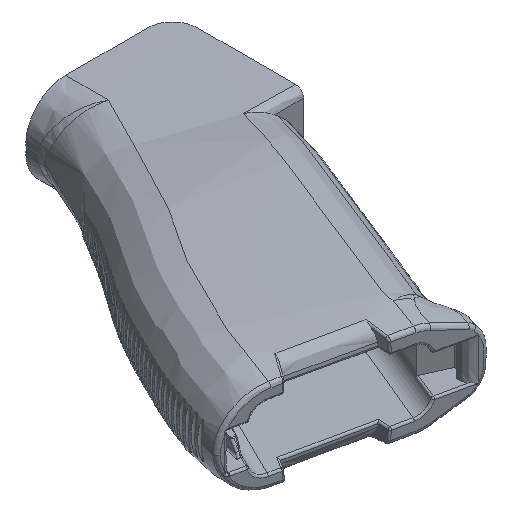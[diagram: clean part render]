
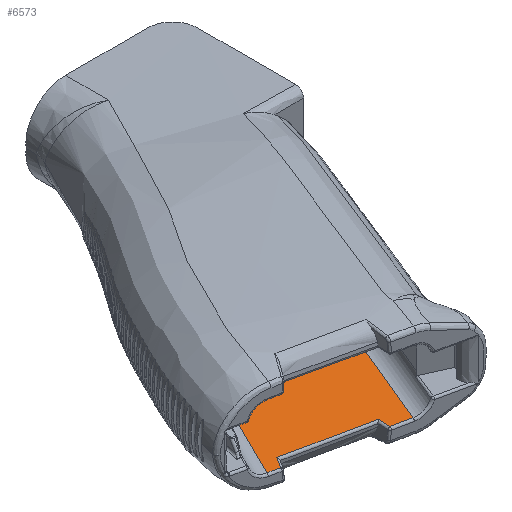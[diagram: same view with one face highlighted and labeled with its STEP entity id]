
A CAD part, isometric view. The second image highlights one B-rep face of the part: STEP entity #6573.
In plain terms, the highlighted planar face has unit normal (-0.007, -0.011, 1).
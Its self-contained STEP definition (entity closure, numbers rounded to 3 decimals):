
#253=PLANE('',#6991);
#409=LINE('',#10048,#641);
#411=LINE('',#10256,#643);
#413=LINE('',#10264,#645);
#414=LINE('',#10269,#646);
#416=LINE('',#10356,#648);
#417=LINE('',#10357,#649);
#641=VECTOR('',#7494,10.);
#643=VECTOR('',#7514,10.);
#645=VECTOR('',#7522,10.);
#646=VECTOR('',#7529,10.);
#648=VECTOR('',#7553,10.);
#649=VECTOR('',#7554,10.);
#950=FACE_OUTER_BOUND('',#1311,.T.);
#1311=EDGE_LOOP('',(#4641,#4642,#4643,#4644,#4645,#4646,#4647,#4648));
#1723=B_SPLINE_CURVE_WITH_KNOTS('',3,(#10187,#10188,#10189,#10190),
 .UNSPECIFIED.,.F.,.F.,(4,4),(-0.294,0.),.UNSPECIFIED.);
#1725=B_SPLINE_CURVE_WITH_KNOTS('',3,(#10296,#10297,#10298,#10299),
 .UNSPECIFIED.,.F.,.F.,(4,4),(-0.488,0.),.UNSPECIFIED.);
#2454=VERTEX_POINT('',#9123);
#2515=VERTEX_POINT('',#10047);
#2518=VERTEX_POINT('',#10185);
#2525=VERTEX_POINT('',#10253);
#2526=VERTEX_POINT('',#10255);
#2529=VERTEX_POINT('',#10263);
#2533=VERTEX_POINT('',#10294);
#2536=VERTEX_POINT('',#10355);
#3336=EDGE_CURVE('',#2454,#2515,#409,.T.);
#3342=EDGE_CURVE('',#2518,#2454,#1723,.T.);
#3349=EDGE_CURVE('',#2525,#2526,#411,.T.);
#3353=EDGE_CURVE('',#2526,#2529,#413,.T.);
#3356=EDGE_CURVE('',#2529,#2518,#414,.T.);
#3360=EDGE_CURVE('',#2533,#2525,#1725,.T.);
#3369=EDGE_CURVE('',#2536,#2533,#416,.T.);
#3370=EDGE_CURVE('',#2515,#2536,#417,.T.);
#4641=ORIENTED_EDGE('',*,*,#3342,.F.);
#4642=ORIENTED_EDGE('',*,*,#3356,.F.);
#4643=ORIENTED_EDGE('',*,*,#3353,.F.);
#4644=ORIENTED_EDGE('',*,*,#3349,.F.);
#4645=ORIENTED_EDGE('',*,*,#3360,.F.);
#4646=ORIENTED_EDGE('',*,*,#3369,.F.);
#4647=ORIENTED_EDGE('',*,*,#3370,.F.);
#4648=ORIENTED_EDGE('',*,*,#3336,.F.);
#6573=ADVANCED_FACE('',(#950),#253,.F.);
#6991=AXIS2_PLACEMENT_3D('',#10354,#7551,#7552);
#7494=DIRECTION('',(0.437,0.9,0.013));
#7514=DIRECTION('',(0.037,0.999,0.012));
#7522=DIRECTION('',(-0.978,0.21,-0.004));
#7529=DIRECTION('',(-0.533,-0.846,-0.013));
#7551=DIRECTION('center_axis',(0.007,0.011,-1.));
#7552=DIRECTION('ref_axis',(-0.865,0.502,0.));
#7553=DIRECTION('',(-0.377,-0.926,-0.013));
#7554=DIRECTION('',(0.865,-0.502,0.));
#9123=CARTESIAN_POINT('',(-202.48,-120.132,-8.381));
#10047=CARTESIAN_POINT('',(-164.577,-42.064,-7.248));
#10048=CARTESIAN_POINT('',(-199.406,-113.8,-8.289));
#10185=CARTESIAN_POINT('',(-199.601,-120.752,-8.369));
#10187=CARTESIAN_POINT('Ctrl Pts',(-199.601,-120.752,
-8.369));
#10188=CARTESIAN_POINT('Ctrl Pts',(-200.561,-120.545,
-8.373));
#10189=CARTESIAN_POINT('Ctrl Pts',(-201.52,-120.339,
-8.377));
#10190=CARTESIAN_POINT('Ctrl Pts',(-202.48,-120.132,
-8.381));
#10253=CARTESIAN_POINT('',(-176.943,-125.629,-8.275));
#10255=CARTESIAN_POINT('',(-176.833,-122.623,-8.241));
#10256=CARTESIAN_POINT('',(-176.678,-118.431,-8.192));
#10263=CARTESIAN_POINT('',(-197.919,-118.083,-8.328));
#10264=CARTESIAN_POINT('',(-192.971,-119.148,-8.307));
#10269=CARTESIAN_POINT('',(-197.515,-117.441,-8.318));
#10294=CARTESIAN_POINT('',(-172.169,-126.657,-8.256));
#10296=CARTESIAN_POINT('Ctrl Pts',(-172.169,-126.657,
-8.256));
#10297=CARTESIAN_POINT('Ctrl Pts',(-173.761,-126.314,
-8.262));
#10298=CARTESIAN_POINT('Ctrl Pts',(-175.352,-125.972,
-8.269));
#10299=CARTESIAN_POINT('Ctrl Pts',(-176.943,-125.629,-8.275));
#10354=CARTESIAN_POINT('Origin',(-207.007,-109.933,-8.295));
#10355=CARTESIAN_POINT('',(-142.87,-54.671,-7.248));
#10356=CARTESIAN_POINT('',(-172.224,-126.791,-8.257));
#10357=CARTESIAN_POINT('',(-160.176,-44.62,-7.248));
